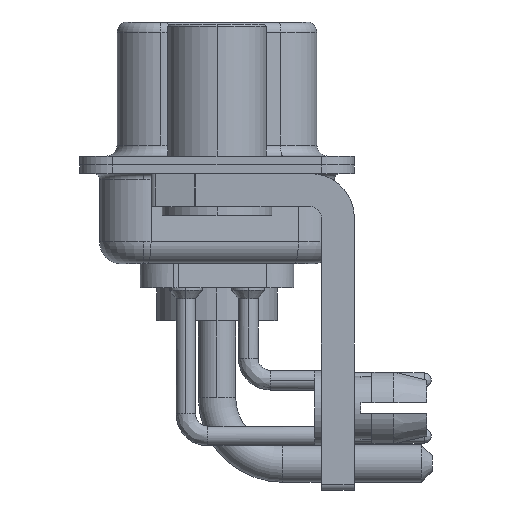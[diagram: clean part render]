
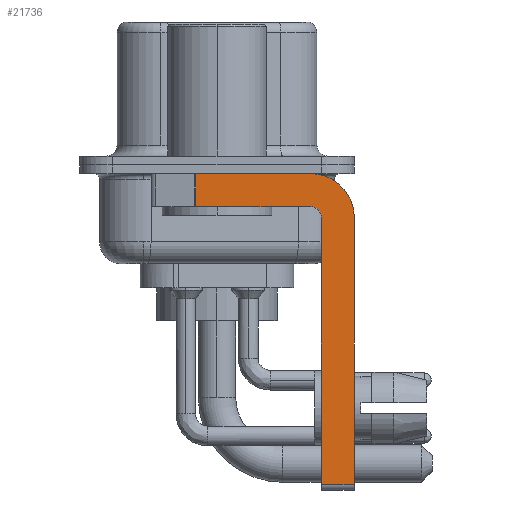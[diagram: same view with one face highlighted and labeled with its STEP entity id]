
A CAD part, left-side view. The second image highlights one B-rep face of the part: STEP entity #21736.
In plain terms, the highlighted planar face has unit normal (-1, 0, 0).
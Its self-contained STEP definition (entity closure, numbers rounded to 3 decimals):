
#293 = ORIENTED_EDGE ( 'NONE', *, *, #13615, .F. ) ;
#357 = LINE ( 'NONE', #3741, #5890 ) ;
#494 = EDGE_CURVE ( 'NONE', #8193, #5914, #21206, .T. ) ;
#642 = VECTOR ( 'NONE', #1277, 1000. ) ;
#686 = VERTEX_POINT ( 'NONE', #19860 ) ;
#1277 = DIRECTION ( 'NONE',  ( 0., 0., -1. ) ) ;
#1307 = CARTESIAN_POINT ( 'NONE',  ( -2.9, 0.978, -1.9 ) ) ;
#1632 = CARTESIAN_POINT ( 'NONE',  ( -2.9, -4.25, -2.4 ) ) ;
#2684 = DIRECTION ( 'NONE',  ( 0., 1., 0. ) ) ;
#2722 = ORIENTED_EDGE ( 'NONE', *, *, #25330, .F. ) ;
#2767 = VECTOR ( 'NONE', #13648, 1000. ) ;
#2934 = CARTESIAN_POINT ( 'NONE',  ( -2.9, -4.25, -1.9 ) ) ;
#3008 = CARTESIAN_POINT ( 'NONE',  ( -2.9, -6.25, -2.4 ) ) ;
#3123 = VERTEX_POINT ( 'NONE', #20993 ) ;
#3598 = LINE ( 'NONE', #19454, #6180 ) ;
#3741 = CARTESIAN_POINT ( 'NONE',  ( -2.9, -4.25, -14.55 ) ) ;
#3743 = EDGE_LOOP ( 'NONE', ( #7348, #19990, #7272, #25163, #293, #20165, #23476, #2722 ) ) ;
#3766 = DIRECTION ( 'NONE',  ( 0., 0., -1. ) ) ;
#3826 = DIRECTION ( 'NONE',  ( 0., 0., 1. ) ) ;
#4206 = DIRECTION ( 'NONE',  ( 0., 0., 1. ) ) ;
#4751 = VERTEX_POINT ( 'NONE', #18336 ) ;
#5770 = FACE_OUTER_BOUND ( 'NONE', #3743, .T. ) ;
#5890 = VECTOR ( 'NONE', #10036, 1000. ) ;
#5914 = VERTEX_POINT ( 'NONE', #11663 ) ;
#6180 = VECTOR ( 'NONE', #23726, 1000. ) ;
#7272 = ORIENTED_EDGE ( 'NONE', *, *, #494, .F. ) ;
#7348 = ORIENTED_EDGE ( 'NONE', *, *, #11320, .F. ) ;
#8193 = VERTEX_POINT ( 'NONE', #2934 ) ;
#9466 = DIRECTION ( 'NONE',  ( 0., 0., -1. ) ) ;
#10036 = DIRECTION ( 'NONE',  ( 0., -1., 0. ) ) ;
#10750 = CARTESIAN_POINT ( 'NONE',  ( -2.9, -4.75, -14.55 ) ) ;
#11320 = EDGE_CURVE ( 'NONE', #4751, #13172, #3598, .T. ) ;
#11663 = CARTESIAN_POINT ( 'NONE',  ( -2.9, 0.978, -1.9 ) ) ;
#11813 = PLANE ( 'NONE',  #18986 ) ;
#11870 = EDGE_CURVE ( 'NONE', #4751, #5914, #13386, .T. ) ;
#12228 = EDGE_CURVE ( 'NONE', #686, #24795, #19649, .T. ) ;
#13172 = VERTEX_POINT ( 'NONE', #18595 ) ;
#13232 = AXIS2_PLACEMENT_3D ( 'NONE', #23946, #15636, #9466 ) ;
#13300 = CARTESIAN_POINT ( 'NONE',  ( -2.9, -4.25, -1.9 ) ) ;
#13386 = LINE ( 'NONE', #1307, #2767 ) ;
#13615 = EDGE_CURVE ( 'NONE', #24343, #3123, #18445, .T. ) ;
#13648 = DIRECTION ( 'NONE',  ( 0., 0., -1. ) ) ;
#13888 = CARTESIAN_POINT ( 'NONE',  ( -2.9, -4.75, -14.8 ) ) ;
#14547 = EDGE_CURVE ( 'NONE', #24343, #24795, #357, .T. ) ;
#15636 = DIRECTION ( 'NONE',  ( 1., 0., 0. ) ) ;
#18336 = CARTESIAN_POINT ( 'NONE',  ( -2.9, 0.978, -0.4 ) ) ;
#18445 = LINE ( 'NONE', #13888, #19983 ) ;
#18595 = CARTESIAN_POINT ( 'NONE',  ( -2.9, -4.25, -0.4 ) ) ;
#18986 = AXIS2_PLACEMENT_3D ( 'NONE', #1632, #22023, #3766 ) ;
#19351 = EDGE_CURVE ( 'NONE', #3123, #8193, #22740, .T. ) ;
#19454 = CARTESIAN_POINT ( 'NONE',  ( -2.9, 3., -0.4 ) ) ;
#19649 = LINE ( 'NONE', #3008, #642 ) ;
#19860 = CARTESIAN_POINT ( 'NONE',  ( -2.9, -6.25, -2.4 ) ) ;
#19983 = VECTOR ( 'NONE', #4206, 1000. ) ;
#19990 = ORIENTED_EDGE ( 'NONE', *, *, #11870, .T. ) ;
#20165 = ORIENTED_EDGE ( 'NONE', *, *, #14547, .T. ) ;
#20325 = DIRECTION ( 'NONE',  ( -1., 0., 0. ) ) ;
#20993 = CARTESIAN_POINT ( 'NONE',  ( -2.9, -4.75, -2.4 ) ) ;
#21206 = LINE ( 'NONE', #13300, #23552 ) ;
#21736 = ADVANCED_FACE ( 'NONE', ( #5770 ), #11813, .F. ) ;
#22023 = DIRECTION ( 'NONE',  ( 1., 0., 0. ) ) ;
#22072 = CARTESIAN_POINT ( 'NONE',  ( -2.9, -4.25, -2.4 ) ) ;
#22740 = CIRCLE ( 'NONE', #25310, 0.5 ) ;
#23476 = ORIENTED_EDGE ( 'NONE', *, *, #12228, .F. ) ;
#23552 = VECTOR ( 'NONE', #2684, 1000. ) ;
#23726 = DIRECTION ( 'NONE',  ( 0., -1., 0. ) ) ;
#23946 = CARTESIAN_POINT ( 'NONE',  ( -2.9, -4.25, -2.4 ) ) ;
#24343 = VERTEX_POINT ( 'NONE', #10750 ) ;
#24795 = VERTEX_POINT ( 'NONE', #25471 ) ;
#25163 = ORIENTED_EDGE ( 'NONE', *, *, #19351, .F. ) ;
#25310 = AXIS2_PLACEMENT_3D ( 'NONE', #22072, #20325, #3826 ) ;
#25330 = EDGE_CURVE ( 'NONE', #13172, #686, #26498, .T. ) ;
#25471 = CARTESIAN_POINT ( 'NONE',  ( -2.9, -6.25, -14.55 ) ) ;
#26498 = CIRCLE ( 'NONE', #13232, 2. ) ;
